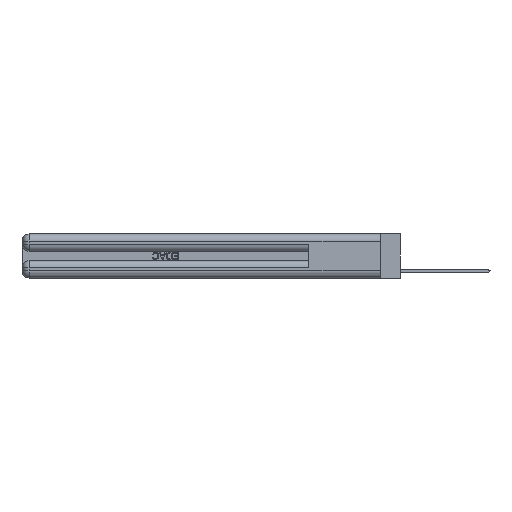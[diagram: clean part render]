
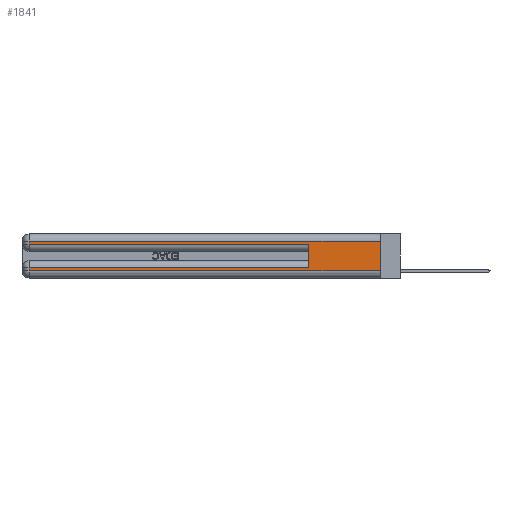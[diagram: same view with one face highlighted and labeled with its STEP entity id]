
A CAD part, left-side view. The second image highlights one B-rep face of the part: STEP entity #1841.
In plain terms, the highlighted planar face has unit normal (-1, 0, 0).
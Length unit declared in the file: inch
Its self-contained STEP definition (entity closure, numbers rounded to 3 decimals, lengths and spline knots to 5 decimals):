
#880 = FACE_OUTER_BOUND ( 'NONE', #19660, .T. ) ;
#1841 = ADVANCED_FACE ( 'NONE', ( #880 ), #11304, .F. ) ;
#2231 = LINE ( 'NONE', #30795, #29496 ) ;
#2271 = VERTEX_POINT ( 'NONE', #19604 ) ;
#2582 = ORIENTED_EDGE ( 'NONE', *, *, #31444, .T. ) ;
#2635 = VERTEX_POINT ( 'NONE', #16501 ) ;
#2899 = ORIENTED_EDGE ( 'NONE', *, *, #23026, .T. ) ;
#3237 = CARTESIAN_POINT ( 'NONE',  ( 0., 2.94, 0.31 ) ) ;
#3508 = ORIENTED_EDGE ( 'NONE', *, *, #20438, .F. ) ;
#3598 = ORIENTED_EDGE ( 'NONE', *, *, #11820, .T. ) ;
#3780 = LINE ( 'NONE', #14559, #23534 ) ;
#4820 = DIRECTION ( 'NONE',  ( 0., 0., 1. ) ) ;
#4906 = EDGE_CURVE ( 'NONE', #10788, #19372, #13196, .T. ) ;
#5268 = CARTESIAN_POINT ( 'NONE',  ( 0., 0., 0.085 ) ) ;
#6537 = ORIENTED_EDGE ( 'NONE', *, *, #4906, .F. ) ;
#6963 = VERTEX_POINT ( 'NONE', #16398 ) ;
#7222 = LINE ( 'NONE', #28090, #25942 ) ;
#8332 = LINE ( 'NONE', #5268, #15321 ) ;
#8363 = DIRECTION ( 'NONE',  ( 0., 0., -1. ) ) ;
#9072 = CARTESIAN_POINT ( 'NONE',  ( 0., 0., 0.37 ) ) ;
#10254 = CARTESIAN_POINT ( 'NONE',  ( 0., 2.94, 0.37 ) ) ;
#10788 = VERTEX_POINT ( 'NONE', #12479 ) ;
#11304 = PLANE ( 'NONE',  #24146 ) ;
#11820 = EDGE_CURVE ( 'NONE', #6963, #14315, #30373, .T. ) ;
#11854 = ORIENTED_EDGE ( 'NONE', *, *, #24312, .T. ) ;
#12104 = CARTESIAN_POINT ( 'NONE',  ( 0., 2.94, 0.085 ) ) ;
#12242 = DIRECTION ( 'NONE',  ( 0., 1., 0. ) ) ;
#12479 = CARTESIAN_POINT ( 'NONE',  ( 0., 0.6, 0.085 ) ) ;
#12976 = EDGE_CURVE ( 'NONE', #14315, #2635, #33694, .T. ) ;
#13196 = LINE ( 'NONE', #25694, #26159 ) ;
#14203 = LINE ( 'NONE', #9072, #31160 ) ;
#14298 = CARTESIAN_POINT ( 'NONE',  ( 0., 0., 0.31 ) ) ;
#14315 = VERTEX_POINT ( 'NONE', #3237 ) ;
#14559 = CARTESIAN_POINT ( 'NONE',  ( 0., 2.94, 0.37 ) ) ;
#15321 = VECTOR ( 'NONE', #31758, 39.37008 ) ;
#16398 = CARTESIAN_POINT ( 'NONE',  ( 0., 0., 0.31 ) ) ;
#16501 = CARTESIAN_POINT ( 'NONE',  ( 0., 2.94, 0.285 ) ) ;
#17218 = ORIENTED_EDGE ( 'NONE', *, *, #22386, .T. ) ;
#18364 = CARTESIAN_POINT ( 'NONE',  ( 0., 0., 0.06 ) ) ;
#19372 = VERTEX_POINT ( 'NONE', #26667 ) ;
#19604 = CARTESIAN_POINT ( 'NONE',  ( 0., 2.94, 0.06 ) ) ;
#19660 = EDGE_LOOP ( 'NONE', ( #3508, #3598, #30724, #11854, #6537, #17218, #2899, #2582 ) ) ;
#20438 = EDGE_CURVE ( 'NONE', #6963, #21429, #14203, .T. ) ;
#21429 = VERTEX_POINT ( 'NONE', #18364 ) ;
#21742 = DIRECTION ( 'NONE',  ( 1., 0., 0. ) ) ;
#22386 = EDGE_CURVE ( 'NONE', #10788, #33609, #8332, .T. ) ;
#23026 = EDGE_CURVE ( 'NONE', #33609, #2271, #3780, .T. ) ;
#23534 = VECTOR ( 'NONE', #25001, 39.37008 ) ;
#24146 = AXIS2_PLACEMENT_3D ( 'NONE', #32504, #21742, #24478 ) ;
#24312 = EDGE_CURVE ( 'NONE', #2635, #19372, #2231, .T. ) ;
#24478 = DIRECTION ( 'NONE',  ( 0., 0., -1. ) ) ;
#25001 = DIRECTION ( 'NONE',  ( 0., 0., -1. ) ) ;
#25694 = CARTESIAN_POINT ( 'NONE',  ( 0., 0.6, 0.145 ) ) ;
#25942 = VECTOR ( 'NONE', #33045, 39.37008 ) ;
#26159 = VECTOR ( 'NONE', #4820, 39.37008 ) ;
#26527 = VECTOR ( 'NONE', #8363, 39.37008 ) ;
#26667 = CARTESIAN_POINT ( 'NONE',  ( 0., 0.6, 0.285 ) ) ;
#28090 = CARTESIAN_POINT ( 'NONE',  ( 0., 0., 0.06 ) ) ;
#28914 = DIRECTION ( 'NONE',  ( 0., -1., 0. ) ) ;
#29496 = VECTOR ( 'NONE', #28914, 39.37008 ) ;
#30279 = DIRECTION ( 'NONE',  ( 0., 0., -1. ) ) ;
#30373 = LINE ( 'NONE', #14298, #30925 ) ;
#30724 = ORIENTED_EDGE ( 'NONE', *, *, #12976, .T. ) ;
#30795 = CARTESIAN_POINT ( 'NONE',  ( 0., 0., 0.285 ) ) ;
#30925 = VECTOR ( 'NONE', #12242, 39.37008 ) ;
#31160 = VECTOR ( 'NONE', #30279, 39.37008 ) ;
#31444 = EDGE_CURVE ( 'NONE', #2271, #21429, #7222, .T. ) ;
#31758 = DIRECTION ( 'NONE',  ( 0., 1., 0. ) ) ;
#32504 = CARTESIAN_POINT ( 'NONE',  ( 0., 0., 0.37 ) ) ;
#33045 = DIRECTION ( 'NONE',  ( 0., -1., 0. ) ) ;
#33609 = VERTEX_POINT ( 'NONE', #12104 ) ;
#33694 = LINE ( 'NONE', #10254, #26527 ) ;
